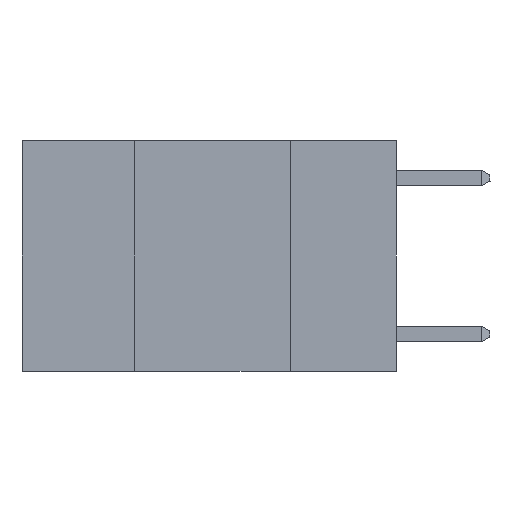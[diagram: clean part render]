
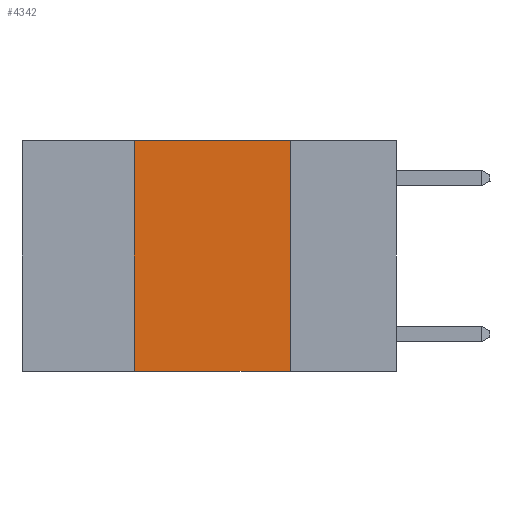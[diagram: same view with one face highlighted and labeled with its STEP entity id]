
A CAD part, left-side view. The second image highlights one B-rep face of the part: STEP entity #4342.
In plain terms, the highlighted planar face has unit normal (-1, 0, 0).
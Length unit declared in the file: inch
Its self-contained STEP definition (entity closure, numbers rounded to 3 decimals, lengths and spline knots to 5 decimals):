
#146 = VERTEX_POINT ( 'NONE', #16539 ) ;
#1137 = VECTOR ( 'NONE', #1593, 39.37008 ) ;
#1593 = DIRECTION ( 'NONE',  ( 0., 0., 1. ) ) ;
#1623 = DIRECTION ( 'NONE',  ( 0., 0., -1. ) ) ;
#2023 = DIRECTION ( 'NONE',  ( 0., 0., -1. ) ) ;
#2056 = LINE ( 'NONE', #6726, #15697 ) ;
#2580 = CARTESIAN_POINT ( 'NONE',  ( 0., 0.6, 0. ) ) ;
#2655 = EDGE_LOOP ( 'NONE', ( #5675, #6123, #6441, #6462 ) ) ;
#3250 = EDGE_CURVE ( 'NONE', #10803, #11744, #12360, .T. ) ;
#3394 = PLANE ( 'NONE',  #5879 ) ;
#3981 = DIRECTION ( 'NONE',  ( 0., -1., 0. ) ) ;
#4342 = ADVANCED_FACE ( 'NONE', ( #15041 ), #3394, .F. ) ;
#5078 = VECTOR ( 'NONE', #1623, 39.37008 ) ;
#5592 = VECTOR ( 'NONE', #3981, 39.37008 ) ;
#5675 = ORIENTED_EDGE ( 'NONE', *, *, #3250, .F. ) ;
#5879 = AXIS2_PLACEMENT_3D ( 'NONE', #6049, #9886, #2023 ) ;
#6049 = CARTESIAN_POINT ( 'NONE',  ( 0., 0.6, 0. ) ) ;
#6123 = ORIENTED_EDGE ( 'NONE', *, *, #16387, .F. ) ;
#6441 = ORIENTED_EDGE ( 'NONE', *, *, #13267, .F. ) ;
#6462 = ORIENTED_EDGE ( 'NONE', *, *, #13239, .T. ) ;
#6726 = CARTESIAN_POINT ( 'NONE',  ( 0., 0.6, -0.37 ) ) ;
#6780 = CARTESIAN_POINT ( 'NONE',  ( 0., 0.42, 0. ) ) ;
#6821 = VERTEX_POINT ( 'NONE', #16030 ) ;
#7988 = DIRECTION ( 'NONE',  ( 0., -1., 0. ) ) ;
#8981 = LINE ( 'NONE', #2580, #5592 ) ;
#9242 = CARTESIAN_POINT ( 'NONE',  ( 0., 0.17, -0.37 ) ) ;
#9546 = CARTESIAN_POINT ( 'NONE',  ( 0., 0.17, 0. ) ) ;
#9886 = DIRECTION ( 'NONE',  ( 1., 0., 0. ) ) ;
#10803 = VERTEX_POINT ( 'NONE', #12380 ) ;
#11744 = VERTEX_POINT ( 'NONE', #9242 ) ;
#12360 = LINE ( 'NONE', #9546, #5078 ) ;
#12380 = CARTESIAN_POINT ( 'NONE',  ( 0., 0.17, 0. ) ) ;
#13239 = EDGE_CURVE ( 'NONE', #6821, #11744, #2056, .T. ) ;
#13267 = EDGE_CURVE ( 'NONE', #6821, #146, #15281, .T. ) ;
#15041 = FACE_OUTER_BOUND ( 'NONE', #2655, .T. ) ;
#15281 = LINE ( 'NONE', #6780, #1137 ) ;
#15697 = VECTOR ( 'NONE', #7988, 39.37008 ) ;
#16030 = CARTESIAN_POINT ( 'NONE',  ( 0., 0.42, -0.37 ) ) ;
#16387 = EDGE_CURVE ( 'NONE', #146, #10803, #8981, .T. ) ;
#16539 = CARTESIAN_POINT ( 'NONE',  ( 0., 0.42, 0. ) ) ;
